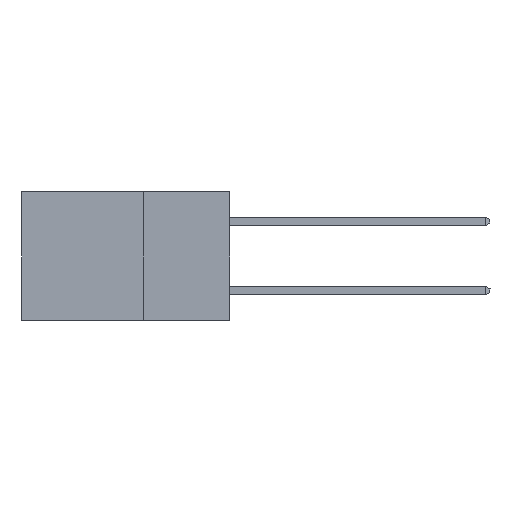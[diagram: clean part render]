
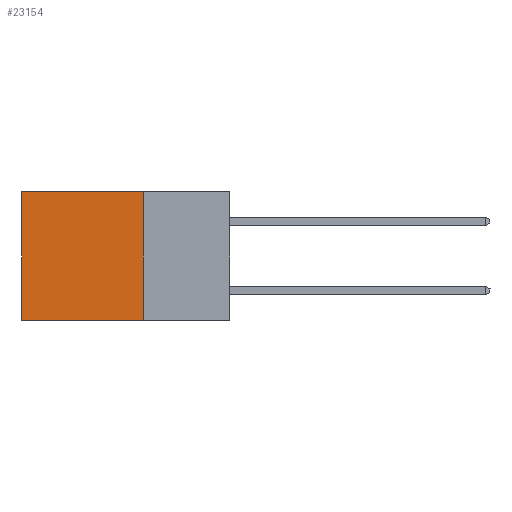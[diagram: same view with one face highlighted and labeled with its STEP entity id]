
A CAD part, left-side view. The second image highlights one B-rep face of the part: STEP entity #23154.
In plain terms, the highlighted planar face has unit normal (-1, 0, 0).
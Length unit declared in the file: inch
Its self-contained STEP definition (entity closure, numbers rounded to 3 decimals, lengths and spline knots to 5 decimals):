
#672 = EDGE_CURVE ( 'NONE', #11616, #25662, #15052, .T. ) ;
#1537 = CARTESIAN_POINT ( 'NONE',  ( 0.2615, 0.25, -0.37 ) ) ;
#1579 = VERTEX_POINT ( 'NONE', #15407 ) ;
#1663 = DIRECTION ( 'NONE',  ( 0., 0., -1. ) ) ;
#1946 = ORIENTED_EDGE ( 'NONE', *, *, #20669, .T. ) ;
#3948 = CARTESIAN_POINT ( 'NONE',  ( 0.2615, 0.6, -0.37 ) ) ;
#4320 = ORIENTED_EDGE ( 'NONE', *, *, #672, .F. ) ;
#5178 = AXIS2_PLACEMENT_3D ( 'NONE', #13140, #21648, #8856 ) ;
#6699 = PLANE ( 'NONE',  #5178 ) ;
#8189 = CARTESIAN_POINT ( 'NONE',  ( 0.2615, 0.25, 0. ) ) ;
#8856 = DIRECTION ( 'NONE',  ( 0., 0., -1. ) ) ;
#9646 = CARTESIAN_POINT ( 'NONE',  ( 0.2615, 0.25, 0. ) ) ;
#11213 = DIRECTION ( 'NONE',  ( 0., 0., -1. ) ) ;
#11234 = VERTEX_POINT ( 'NONE', #3948 ) ;
#11616 = VERTEX_POINT ( 'NONE', #8189 ) ;
#13027 = LINE ( 'NONE', #22147, #23608 ) ;
#13140 = CARTESIAN_POINT ( 'NONE',  ( 0.2615, 0.25, -0.37 ) ) ;
#14847 = VECTOR ( 'NONE', #18301, 39.37008 ) ;
#15052 = LINE ( 'NONE', #1537, #20653 ) ;
#15407 = CARTESIAN_POINT ( 'NONE',  ( 0.2615, 0.6, 0. ) ) ;
#15979 = EDGE_LOOP ( 'NONE', ( #21466, #25380, #4320, #1946 ) ) ;
#16837 = EDGE_CURVE ( 'NONE', #1579, #11234, #21948, .T. ) ;
#16964 = EDGE_CURVE ( 'NONE', #25662, #11234, #13027, .T. ) ;
#18277 = CARTESIAN_POINT ( 'NONE',  ( 0.2615, 0.25, -0.37 ) ) ;
#18301 = DIRECTION ( 'NONE',  ( 0., 1., 0. ) ) ;
#20653 = VECTOR ( 'NONE', #1663, 39.37008 ) ;
#20669 = EDGE_CURVE ( 'NONE', #11616, #1579, #26037, .T. ) ;
#21466 = ORIENTED_EDGE ( 'NONE', *, *, #16837, .T. ) ;
#21648 = DIRECTION ( 'NONE',  ( 1., 0., 0. ) ) ;
#21948 = LINE ( 'NONE', #23823, #26853 ) ;
#22147 = CARTESIAN_POINT ( 'NONE',  ( 0.2615, 0.25, -0.37 ) ) ;
#23154 = ADVANCED_FACE ( 'NONE', ( #23619 ), #6699, .F. ) ;
#23608 = VECTOR ( 'NONE', #24268, 39.37008 ) ;
#23619 = FACE_OUTER_BOUND ( 'NONE', #15979, .T. ) ;
#23823 = CARTESIAN_POINT ( 'NONE',  ( 0.2615, 0.6, -0.37 ) ) ;
#24268 = DIRECTION ( 'NONE',  ( 0., 1., 0. ) ) ;
#25380 = ORIENTED_EDGE ( 'NONE', *, *, #16964, .F. ) ;
#25662 = VERTEX_POINT ( 'NONE', #18277 ) ;
#26037 = LINE ( 'NONE', #9646, #14847 ) ;
#26853 = VECTOR ( 'NONE', #11213, 39.37008 ) ;
